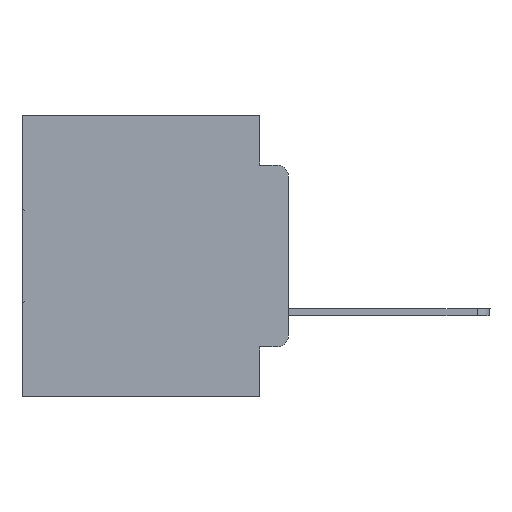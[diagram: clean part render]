
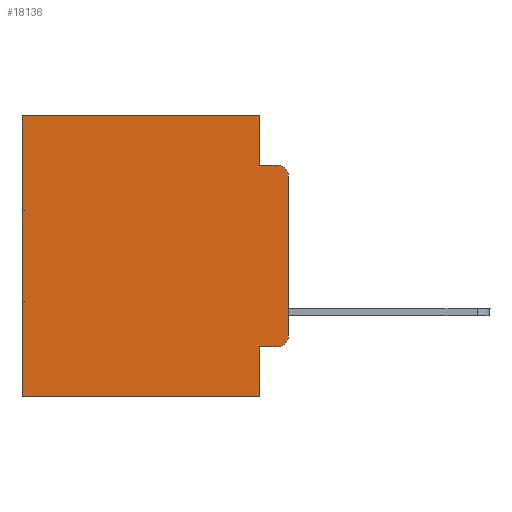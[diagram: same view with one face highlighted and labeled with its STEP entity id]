
A CAD part, left-side view. The second image highlights one B-rep face of the part: STEP entity #18136.
In plain terms, the highlighted planar face has unit normal (-1, 0, 0).
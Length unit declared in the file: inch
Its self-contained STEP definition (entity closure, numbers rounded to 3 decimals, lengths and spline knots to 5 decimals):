
#300 = CARTESIAN_POINT ( 'NONE',  ( 0.298, 0.051, 0. ) ) ;
#344 = CARTESIAN_POINT ( 'NONE',  ( 0.298, 0.473, -0.5 ) ) ;
#393 = LINE ( 'NONE', #14838, #26340 ) ;
#412 = EDGE_CURVE ( 'NONE', #8725, #10194, #27267, .T. ) ;
#553 = VERTEX_POINT ( 'NONE', #6184 ) ;
#905 = DIRECTION ( 'NONE',  ( 0., -1., 0. ) ) ;
#2847 = CARTESIAN_POINT ( 'NONE',  ( 0.298, 0.051, -0.4115 ) ) ;
#2975 = EDGE_CURVE ( 'NONE', #24830, #24715, #20651, .T. ) ;
#3291 = CARTESIAN_POINT ( 'NONE',  ( 0.298, 0.02, -0.3915 ) ) ;
#3476 = ORIENTED_EDGE ( 'NONE', *, *, #18962, .F. ) ;
#3497 = VECTOR ( 'NONE', #21985, 39.37008 ) ;
#4708 = ORIENTED_EDGE ( 'NONE', *, *, #2975, .T. ) ;
#5120 = LINE ( 'NONE', #15005, #3497 ) ;
#5621 = EDGE_CURVE ( 'NONE', #16372, #13106, #5120, .T. ) ;
#6184 = CARTESIAN_POINT ( 'NONE',  ( 0.298, 0.051, -0.0885 ) ) ;
#7818 = CARTESIAN_POINT ( 'NONE',  ( 0.298, 0., 0. ) ) ;
#8092 = VERTEX_POINT ( 'NONE', #11266 ) ;
#8288 = PLANE ( 'NONE',  #24819 ) ;
#8318 = DIRECTION ( 'NONE',  ( 0., 0., -1. ) ) ;
#8462 = CARTESIAN_POINT ( 'NONE',  ( 0.298, 0.02, -0.4115 ) ) ;
#8636 = DIRECTION ( 'NONE',  ( -1., 0., 0. ) ) ;
#8668 = LINE ( 'NONE', #16137, #28186 ) ;
#8725 = VERTEX_POINT ( 'NONE', #12940 ) ;
#8816 = DIRECTION ( 'NONE',  ( 0., 1., 0. ) ) ;
#9105 = CARTESIAN_POINT ( 'NONE',  ( 0.298, 0.051, -0.4115 ) ) ;
#10066 = DIRECTION ( 'NONE',  ( 0., 0., -1. ) ) ;
#10167 = EDGE_CURVE ( 'NONE', #24715, #10194, #11424, .T. ) ;
#10194 = VERTEX_POINT ( 'NONE', #13316 ) ;
#10248 = DIRECTION ( 'NONE',  ( 0., 0., -1. ) ) ;
#10424 = LINE ( 'NONE', #20324, #31055 ) ;
#10699 = CARTESIAN_POINT ( 'NONE',  ( 0.298, 0., 0. ) ) ;
#10894 = ORIENTED_EDGE ( 'NONE', *, *, #17700, .F. ) ;
#11073 = EDGE_LOOP ( 'NONE', ( #15384, #31810, #14956, #31283, #24617, #13841, #3476, #10894, #4708, #21557 ) ) ;
#11195 = DIRECTION ( 'NONE',  ( 0., 0., -1. ) ) ;
#11247 = DIRECTION ( 'NONE',  ( 0., -1., 0. ) ) ;
#11266 = CARTESIAN_POINT ( 'NONE',  ( 0.298, 0.051, -0.5 ) ) ;
#11424 = CIRCLE ( 'NONE', #15586, 0.02 ) ;
#11890 = EDGE_CURVE ( 'NONE', #20791, #553, #29798, .T. ) ;
#12055 = VECTOR ( 'NONE', #20055, 39.37008 ) ;
#12940 = CARTESIAN_POINT ( 'NONE',  ( 0.298, 0., -0.1085 ) ) ;
#13106 = VERTEX_POINT ( 'NONE', #344 ) ;
#13143 = DIRECTION ( 'NONE',  ( 1., 0., 0. ) ) ;
#13316 = CARTESIAN_POINT ( 'NONE',  ( 0.298, 0., -0.3915 ) ) ;
#13742 = CARTESIAN_POINT ( 'NONE',  ( 0.298, 0., 0. ) ) ;
#13801 = FACE_OUTER_BOUND ( 'NONE', #11073, .T. ) ;
#13841 = ORIENTED_EDGE ( 'NONE', *, *, #5621, .T. ) ;
#14838 = CARTESIAN_POINT ( 'NONE',  ( 0.298, 0.051, 0. ) ) ;
#14851 = CIRCLE ( 'NONE', #22572, 0.02 ) ;
#14956 = ORIENTED_EDGE ( 'NONE', *, *, #26264, .F. ) ;
#15005 = CARTESIAN_POINT ( 'NONE',  ( 0.298, 0.473, 0. ) ) ;
#15384 = ORIENTED_EDGE ( 'NONE', *, *, #412, .F. ) ;
#15586 = AXIS2_PLACEMENT_3D ( 'NONE', #3291, #28558, #11195 ) ;
#15939 = CARTESIAN_POINT ( 'NONE',  ( 0.298, 0.02, -0.1085 ) ) ;
#16137 = CARTESIAN_POINT ( 'NONE',  ( 0.298, 0.051, -0.0885 ) ) ;
#16372 = VERTEX_POINT ( 'NONE', #30191 ) ;
#16510 = EDGE_CURVE ( 'NONE', #8725, #26873, #14851, .T. ) ;
#17411 = VECTOR ( 'NONE', #31387, 39.37008 ) ;
#17700 = EDGE_CURVE ( 'NONE', #24830, #8092, #393, .T. ) ;
#18136 = ADVANCED_FACE ( 'NONE', ( #13801 ), #8288, .F. ) ;
#18962 = EDGE_CURVE ( 'NONE', #8092, #13106, #10424, .T. ) ;
#19292 = CARTESIAN_POINT ( 'NONE',  ( 0.298, 0.02, -0.0885 ) ) ;
#19513 = CARTESIAN_POINT ( 'NONE',  ( 0.298, 0.051, 0. ) ) ;
#20055 = DIRECTION ( 'NONE',  ( 0., 0., -1. ) ) ;
#20324 = CARTESIAN_POINT ( 'NONE',  ( 0.298, 0., -0.5 ) ) ;
#20651 = LINE ( 'NONE', #2847, #25776 ) ;
#20791 = VERTEX_POINT ( 'NONE', #19513 ) ;
#21182 = LINE ( 'NONE', #13742, #17411 ) ;
#21557 = ORIENTED_EDGE ( 'NONE', *, *, #10167, .T. ) ;
#21977 = VECTOR ( 'NONE', #10066, 39.37008 ) ;
#21985 = DIRECTION ( 'NONE',  ( 0., 0., -1. ) ) ;
#22572 = AXIS2_PLACEMENT_3D ( 'NONE', #15939, #8636, #8318 ) ;
#24617 = ORIENTED_EDGE ( 'NONE', *, *, #28050, .T. ) ;
#24715 = VERTEX_POINT ( 'NONE', #8462 ) ;
#24819 = AXIS2_PLACEMENT_3D ( 'NONE', #10699, #13143, #25632 ) ;
#24830 = VERTEX_POINT ( 'NONE', #9105 ) ;
#25632 = DIRECTION ( 'NONE',  ( 0., 0., -1. ) ) ;
#25776 = VECTOR ( 'NONE', #905, 39.37008 ) ;
#26264 = EDGE_CURVE ( 'NONE', #553, #26873, #8668, .T. ) ;
#26340 = VECTOR ( 'NONE', #10248, 39.37008 ) ;
#26873 = VERTEX_POINT ( 'NONE', #19292 ) ;
#27267 = LINE ( 'NONE', #7818, #21977 ) ;
#28050 = EDGE_CURVE ( 'NONE', #20791, #16372, #21182, .T. ) ;
#28186 = VECTOR ( 'NONE', #11247, 39.37008 ) ;
#28558 = DIRECTION ( 'NONE',  ( -1., 0., 0. ) ) ;
#29798 = LINE ( 'NONE', #300, #12055 ) ;
#30191 = CARTESIAN_POINT ( 'NONE',  ( 0.298, 0.473, 0. ) ) ;
#31055 = VECTOR ( 'NONE', #8816, 39.37008 ) ;
#31283 = ORIENTED_EDGE ( 'NONE', *, *, #11890, .F. ) ;
#31387 = DIRECTION ( 'NONE',  ( 0., 1., 0. ) ) ;
#31810 = ORIENTED_EDGE ( 'NONE', *, *, #16510, .T. ) ;
